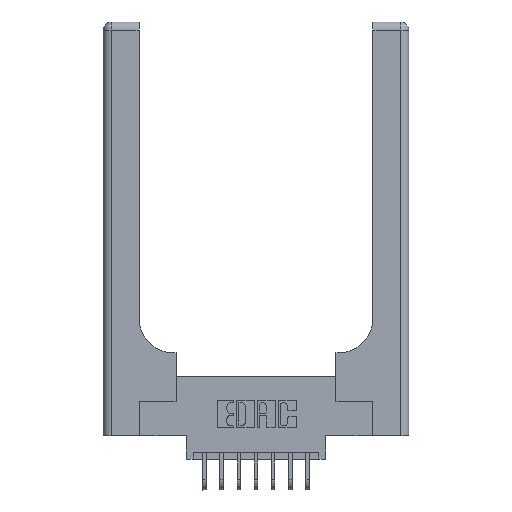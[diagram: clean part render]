
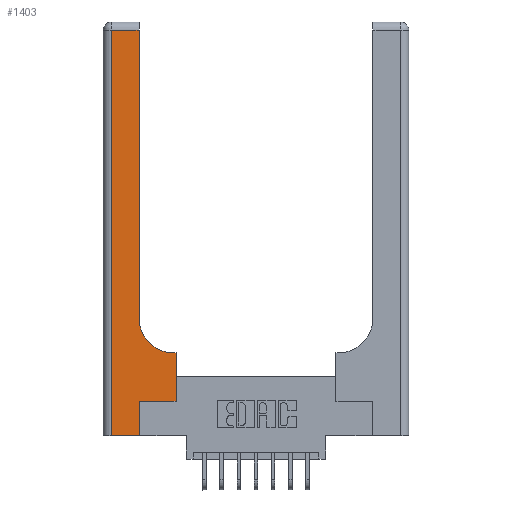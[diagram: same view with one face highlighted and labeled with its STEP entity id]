
A CAD part, top view. The second image highlights one B-rep face of the part: STEP entity #1403.
In plain terms, the highlighted planar face has unit normal (0, 0, 1).
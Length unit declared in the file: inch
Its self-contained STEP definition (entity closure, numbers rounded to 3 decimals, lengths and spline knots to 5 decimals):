
#82 = VECTOR ( 'NONE', #2445, 39.37008 ) ;
#304 = CARTESIAN_POINT ( 'NONE',  ( 0.265, 0., 0.37 ) ) ;
#1124 = CARTESIAN_POINT ( 'NONE',  ( 0.26, 0.85, 0.37 ) ) ;
#1141 = LINE ( 'NONE', #14865, #2146 ) ;
#1235 = VECTOR ( 'NONE', #7935, 39.37008 ) ;
#1403 = ADVANCED_FACE ( 'NONE', ( #6306 ), #5374, .F. ) ;
#1541 = VERTEX_POINT ( 'NONE', #15839 ) ;
#1572 = CARTESIAN_POINT ( 'NONE',  ( 0.06, 0., 0.37 ) ) ;
#1601 = VECTOR ( 'NONE', #10988, 39.37008 ) ;
#2146 = VECTOR ( 'NONE', #8498, 39.37008 ) ;
#2165 = DIRECTION ( 'NONE',  ( 1., 0., 0. ) ) ;
#2209 = EDGE_LOOP ( 'NONE', ( #2964, #4695, #4544, #12724, #12539, #4904, #11300, #7428, #2931 ) ) ;
#2445 = DIRECTION ( 'NONE',  ( 0., 1., 0. ) ) ;
#2665 = LINE ( 'NONE', #9318, #14200 ) ;
#2931 = ORIENTED_EDGE ( 'NONE', *, *, #9051, .T. ) ;
#2964 = ORIENTED_EDGE ( 'NONE', *, *, #9314, .T. ) ;
#3232 = LINE ( 'NONE', #4221, #1235 ) ;
#3826 = EDGE_CURVE ( 'NONE', #10000, #3913, #3232, .T. ) ;
#3913 = VERTEX_POINT ( 'NONE', #9501 ) ;
#4066 = DIRECTION ( 'NONE',  ( 0., 0., -1. ) ) ;
#4221 = CARTESIAN_POINT ( 'NONE',  ( 0.265, 0., 0.37 ) ) ;
#4382 = LINE ( 'NONE', #9317, #1601 ) ;
#4544 = ORIENTED_EDGE ( 'NONE', *, *, #11419, .T. ) ;
#4617 = DIRECTION ( 'NONE',  ( 0., 0., -1. ) ) ;
#4695 = ORIENTED_EDGE ( 'NONE', *, *, #14182, .T. ) ;
#4904 = ORIENTED_EDGE ( 'NONE', *, *, #14898, .T. ) ;
#5374 = PLANE ( 'NONE',  #13951 ) ;
#5567 = VECTOR ( 'NONE', #9889, 39.37008 ) ;
#5917 = DIRECTION ( 'NONE',  ( 1., 0., 0. ) ) ;
#5938 = CARTESIAN_POINT ( 'NONE',  ( 0., 2.94, 0.37 ) ) ;
#6306 = FACE_OUTER_BOUND ( 'NONE', #2209, .T. ) ;
#6753 = VERTEX_POINT ( 'NONE', #14217 ) ;
#7071 = VERTEX_POINT ( 'NONE', #11117 ) ;
#7072 = VERTEX_POINT ( 'NONE', #13666 ) ;
#7428 = ORIENTED_EDGE ( 'NONE', *, *, #8275, .T. ) ;
#7665 = CARTESIAN_POINT ( 'NONE',  ( 0.26, 2.94, 0.37 ) ) ;
#7935 = DIRECTION ( 'NONE',  ( 0., 1., 0. ) ) ;
#8275 = EDGE_CURVE ( 'NONE', #7072, #6753, #2665, .T. ) ;
#8498 = DIRECTION ( 'NONE',  ( 0., 1., 0. ) ) ;
#8942 = LINE ( 'NONE', #5938, #5567 ) ;
#9051 = EDGE_CURVE ( 'NONE', #6753, #12353, #13382, .T. ) ;
#9150 = CARTESIAN_POINT ( 'NONE',  ( 0., 3., 0.37 ) ) ;
#9314 = EDGE_CURVE ( 'NONE', #12353, #15173, #15345, .T. ) ;
#9317 = CARTESIAN_POINT ( 'NONE',  ( 0.06, 3., 0.37 ) ) ;
#9318 = CARTESIAN_POINT ( 'NONE',  ( 0.26, 0.6, 0.37 ) ) ;
#9501 = CARTESIAN_POINT ( 'NONE',  ( 0.265, 0.25, 0.37 ) ) ;
#9506 = VECTOR ( 'NONE', #5917, 39.37008 ) ;
#9757 = CARTESIAN_POINT ( 'NONE',  ( 0., 0., 0.37 ) ) ;
#9889 = DIRECTION ( 'NONE',  ( -1., 0., 0. ) ) ;
#10000 = VERTEX_POINT ( 'NONE', #304 ) ;
#10428 = AXIS2_PLACEMENT_3D ( 'NONE', #10908, #4617, #13544 ) ;
#10491 = LINE ( 'NONE', #16150, #9506 ) ;
#10643 = DIRECTION ( 'NONE',  ( -1., 0., 0. ) ) ;
#10908 = CARTESIAN_POINT ( 'NONE',  ( 0.51, 0.85, 0.37 ) ) ;
#10988 = DIRECTION ( 'NONE',  ( 0., -1., 0. ) ) ;
#11117 = CARTESIAN_POINT ( 'NONE',  ( 0.06, 2.94, 0.37 ) ) ;
#11300 = ORIENTED_EDGE ( 'NONE', *, *, #15201, .T. ) ;
#11419 = EDGE_CURVE ( 'NONE', #7071, #15066, #4382, .T. ) ;
#11471 = CARTESIAN_POINT ( 'NONE',  ( 0.26, 3., 0.37 ) ) ;
#12353 = VERTEX_POINT ( 'NONE', #1124 ) ;
#12539 = ORIENTED_EDGE ( 'NONE', *, *, #3826, .T. ) ;
#12724 = ORIENTED_EDGE ( 'NONE', *, *, #14044, .T. ) ;
#12757 = LINE ( 'NONE', #9757, #16149 ) ;
#13382 = CIRCLE ( 'NONE', #10428, 0.25 ) ;
#13544 = DIRECTION ( 'NONE',  ( 1., 0., 0. ) ) ;
#13666 = CARTESIAN_POINT ( 'NONE',  ( 0.528, 0.6, 0.37 ) ) ;
#13951 = AXIS2_PLACEMENT_3D ( 'NONE', #9150, #4066, #15406 ) ;
#14044 = EDGE_CURVE ( 'NONE', #15066, #10000, #12757, .T. ) ;
#14182 = EDGE_CURVE ( 'NONE', #15173, #7071, #8942, .T. ) ;
#14200 = VECTOR ( 'NONE', #10643, 39.37008 ) ;
#14217 = CARTESIAN_POINT ( 'NONE',  ( 0.51, 0.6, 0.37 ) ) ;
#14865 = CARTESIAN_POINT ( 'NONE',  ( 0.528, 0.25, 0.37 ) ) ;
#14898 = EDGE_CURVE ( 'NONE', #3913, #1541, #10491, .T. ) ;
#15066 = VERTEX_POINT ( 'NONE', #1572 ) ;
#15173 = VERTEX_POINT ( 'NONE', #7665 ) ;
#15201 = EDGE_CURVE ( 'NONE', #1541, #7072, #1141, .T. ) ;
#15345 = LINE ( 'NONE', #11471, #82 ) ;
#15406 = DIRECTION ( 'NONE',  ( -1., 0., 0. ) ) ;
#15839 = CARTESIAN_POINT ( 'NONE',  ( 0.528, 0.25, 0.37 ) ) ;
#16149 = VECTOR ( 'NONE', #2165, 39.37008 ) ;
#16150 = CARTESIAN_POINT ( 'NONE',  ( 0.265, 0.25, 0.37 ) ) ;
